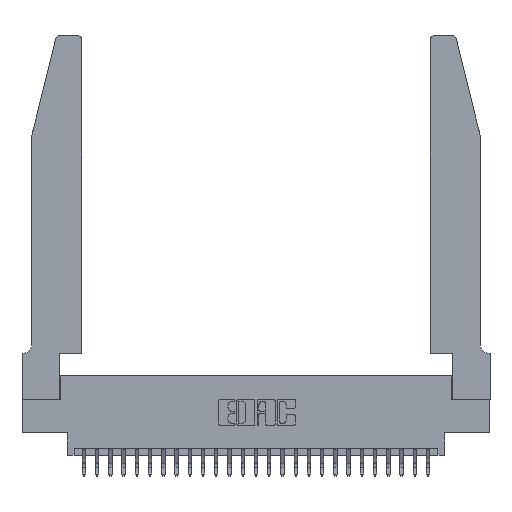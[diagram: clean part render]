
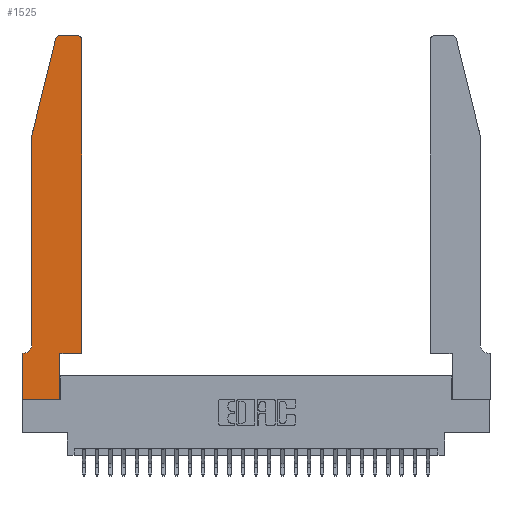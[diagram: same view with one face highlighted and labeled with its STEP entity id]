
A CAD part, top view. The second image highlights one B-rep face of the part: STEP entity #1525.
In plain terms, the highlighted planar face has unit normal (0, 0, 1).
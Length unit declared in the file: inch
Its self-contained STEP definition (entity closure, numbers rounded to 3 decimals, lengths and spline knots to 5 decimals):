
#202 = VECTOR ( 'NONE', #3828, 39.37008 ) ;
#679 = ORIENTED_EDGE ( 'NONE', *, *, #7551, .T. ) ;
#1124 = VERTEX_POINT ( 'NONE', #12718 ) ;
#1334 = LINE ( 'NONE', #5323, #12350 ) ;
#1494 = EDGE_CURVE ( 'NONE', #20837, #23758, #4218, .T. ) ;
#1525 = ADVANCED_FACE ( 'NONE', ( #20323 ), #16130, .T. ) ;
#1632 = CARTESIAN_POINT ( 'NONE',  ( 0.4505, 0.35, 0.37 ) ) ;
#2205 = EDGE_CURVE ( 'NONE', #28009, #13888, #9659, .T. ) ;
#2281 = EDGE_CURVE ( 'NONE', #4741, #21349, #12612, .T. ) ;
#2833 = VECTOR ( 'NONE', #8932, 39.37008 ) ;
#3094 = ORIENTED_EDGE ( 'NONE', *, *, #12551, .T. ) ;
#3449 = CARTESIAN_POINT ( 'NONE',  ( 0.25487, 2.72718, 0.37 ) ) ;
#3468 = DIRECTION ( 'NONE',  ( 1., 0., 0. ) ) ;
#3644 = CARTESIAN_POINT ( 'NONE',  ( 0.0055, 0.42, 0.37 ) ) ;
#3828 = DIRECTION ( 'NONE',  ( -0.239, -0.971, 0. ) ) ;
#3830 = VECTOR ( 'NONE', #25149, 39.37008 ) ;
#4218 = LINE ( 'NONE', #11648, #10051 ) ;
#4480 = ORIENTED_EDGE ( 'NONE', *, *, #8691, .T. ) ;
#4741 = VERTEX_POINT ( 'NONE', #3449 ) ;
#5027 = VERTEX_POINT ( 'NONE', #8837 ) ;
#5323 = CARTESIAN_POINT ( 'NONE',  ( 0.2865, 0.35, 0.37 ) ) ;
#5504 = CARTESIAN_POINT ( 'NONE',  ( 0.2605, 2.75, 0.37 ) ) ;
#5733 = VECTOR ( 'NONE', #3468, 39.37008 ) ;
#5810 = LINE ( 'NONE', #5504, #11654 ) ;
#5851 = DIRECTION ( 'NONE',  ( -1., 0., 0. ) ) ;
#6547 = ORIENTED_EDGE ( 'NONE', *, *, #1494, .T. ) ;
#6815 = CARTESIAN_POINT ( 'NONE',  ( 0.0755, 0.35, 0.37 ) ) ;
#7043 = CARTESIAN_POINT ( 'NONE',  ( 0., 0., 0.37 ) ) ;
#7528 = CIRCLE ( 'NONE', #15624, 0.03 ) ;
#7551 = EDGE_CURVE ( 'NONE', #16499, #20837, #1334, .T. ) ;
#7576 = EDGE_CURVE ( 'NONE', #21167, #10821, #5810, .T. ) ;
#7698 = ORIENTED_EDGE ( 'NONE', *, *, #21285, .T. ) ;
#8149 = CARTESIAN_POINT ( 'NONE',  ( 0.0755, 2., 0.37 ) ) ;
#8691 = EDGE_CURVE ( 'NONE', #5027, #28009, #20326, .T. ) ;
#8837 = CARTESIAN_POINT ( 'NONE',  ( 0.0055, 0.35, 0.37 ) ) ;
#8932 = DIRECTION ( 'NONE',  ( -1., 0., 0. ) ) ;
#8994 = DIRECTION ( 'NONE',  ( 0., 1., 0. ) ) ;
#9630 = EDGE_CURVE ( 'NONE', #1124, #21167, #13783, .T. ) ;
#9659 = LINE ( 'NONE', #16399, #3830 ) ;
#10051 = VECTOR ( 'NONE', #22537, 39.37008 ) ;
#10405 = DIRECTION ( 'NONE',  ( 0., 0., 1. ) ) ;
#10599 = CARTESIAN_POINT ( 'NONE',  ( 0.0755, 0.42, 0.37 ) ) ;
#10770 = EDGE_LOOP ( 'NONE', ( #13407, #24987, #25680, #3094, #21272, #4480, #11026, #7698, #679, #6547, #24004, #18892 ) ) ;
#10821 = VERTEX_POINT ( 'NONE', #27690 ) ;
#11026 = ORIENTED_EDGE ( 'NONE', *, *, #2205, .T. ) ;
#11061 = LINE ( 'NONE', #24357, #27746 ) ;
#11587 = LINE ( 'NONE', #20817, #5733 ) ;
#11639 = DIRECTION ( 'NONE',  ( 0., 0., 1. ) ) ;
#11648 = CARTESIAN_POINT ( 'NONE',  ( 0.4505, 0.35, 0.37 ) ) ;
#11654 = VECTOR ( 'NONE', #20848, 39.37008 ) ;
#12143 = CARTESIAN_POINT ( 'NONE',  ( 0.0755, 2., 0.37 ) ) ;
#12350 = VECTOR ( 'NONE', #22858, 39.37008 ) ;
#12551 = EDGE_CURVE ( 'NONE', #21349, #17856, #22495, .T. ) ;
#12612 = LINE ( 'NONE', #8149, #202 ) ;
#12718 = CARTESIAN_POINT ( 'NONE',  ( 0.4505, 2.72, 0.37 ) ) ;
#12879 = CARTESIAN_POINT ( 'NONE',  ( 0.2865, 0., 0.37 ) ) ;
#13017 = CIRCLE ( 'NONE', #18871, 0.07 ) ;
#13407 = ORIENTED_EDGE ( 'NONE', *, *, #7576, .T. ) ;
#13783 = CIRCLE ( 'NONE', #17411, 0.03 ) ;
#13888 = VERTEX_POINT ( 'NONE', #7043 ) ;
#13946 = CARTESIAN_POINT ( 'NONE',  ( 0., 0.35, 0.37 ) ) ;
#13948 = CARTESIAN_POINT ( 'NONE',  ( 0.4205, 2.75, 0.37 ) ) ;
#14964 = AXIS2_PLACEMENT_3D ( 'NONE', #13946, #22629, #18329 ) ;
#15624 = AXIS2_PLACEMENT_3D ( 'NONE', #24683, #11639, #26880 ) ;
#16130 = PLANE ( 'NONE',  #14964 ) ;
#16399 = CARTESIAN_POINT ( 'NONE',  ( 0., 0., 0.37 ) ) ;
#16499 = VERTEX_POINT ( 'NONE', #12879 ) ;
#16696 = VECTOR ( 'NONE', #22497, 39.37008 ) ;
#17411 = AXIS2_PLACEMENT_3D ( 'NONE', #23512, #10405, #25661 ) ;
#17856 = VERTEX_POINT ( 'NONE', #10599 ) ;
#18329 = DIRECTION ( 'NONE',  ( 1., 0., 0. ) ) ;
#18568 = EDGE_CURVE ( 'NONE', #23758, #1124, #11061, .T. ) ;
#18871 = AXIS2_PLACEMENT_3D ( 'NONE', #3644, #18983, #5851 ) ;
#18892 = ORIENTED_EDGE ( 'NONE', *, *, #9630, .T. ) ;
#18983 = DIRECTION ( 'NONE',  ( 0., 0., -1. ) ) ;
#19405 = CARTESIAN_POINT ( 'NONE',  ( 0., 0.35, 0.37 ) ) ;
#20302 = CARTESIAN_POINT ( 'NONE',  ( 0.0755, 2., 0.37 ) ) ;
#20323 = FACE_OUTER_BOUND ( 'NONE', #10770, .T. ) ;
#20326 = LINE ( 'NONE', #6815, #2833 ) ;
#20817 = CARTESIAN_POINT ( 'NONE',  ( 0., 0., 0.37 ) ) ;
#20837 = VERTEX_POINT ( 'NONE', #21603 ) ;
#20848 = DIRECTION ( 'NONE',  ( -1., 0., 0. ) ) ;
#21167 = VERTEX_POINT ( 'NONE', #13948 ) ;
#21272 = ORIENTED_EDGE ( 'NONE', *, *, #21924, .T. ) ;
#21285 = EDGE_CURVE ( 'NONE', #13888, #16499, #11587, .T. ) ;
#21349 = VERTEX_POINT ( 'NONE', #12143 ) ;
#21603 = CARTESIAN_POINT ( 'NONE',  ( 0.2865, 0.35, 0.37 ) ) ;
#21924 = EDGE_CURVE ( 'NONE', #17856, #5027, #13017, .T. ) ;
#22495 = LINE ( 'NONE', #20302, #16696 ) ;
#22497 = DIRECTION ( 'NONE',  ( 0., -1., 0. ) ) ;
#22537 = DIRECTION ( 'NONE',  ( 1., 0., 0. ) ) ;
#22629 = DIRECTION ( 'NONE',  ( 0., 0., 1. ) ) ;
#22858 = DIRECTION ( 'NONE',  ( 0., 1., 0. ) ) ;
#23512 = CARTESIAN_POINT ( 'NONE',  ( 0.4205, 2.72, 0.37 ) ) ;
#23758 = VERTEX_POINT ( 'NONE', #1632 ) ;
#24004 = ORIENTED_EDGE ( 'NONE', *, *, #18568, .T. ) ;
#24357 = CARTESIAN_POINT ( 'NONE',  ( 0.4505, 0.35, 0.37 ) ) ;
#24683 = CARTESIAN_POINT ( 'NONE',  ( 0.284, 2.72, 0.37 ) ) ;
#24987 = ORIENTED_EDGE ( 'NONE', *, *, #28271, .T. ) ;
#25149 = DIRECTION ( 'NONE',  ( 0., -1., 0. ) ) ;
#25661 = DIRECTION ( 'NONE',  ( 1., 0., 0. ) ) ;
#25680 = ORIENTED_EDGE ( 'NONE', *, *, #2281, .T. ) ;
#26880 = DIRECTION ( 'NONE',  ( 1., 0., 0. ) ) ;
#27690 = CARTESIAN_POINT ( 'NONE',  ( 0.284, 2.75, 0.37 ) ) ;
#27746 = VECTOR ( 'NONE', #8994, 39.37008 ) ;
#28009 = VERTEX_POINT ( 'NONE', #19405 ) ;
#28271 = EDGE_CURVE ( 'NONE', #10821, #4741, #7528, .T. ) ;
